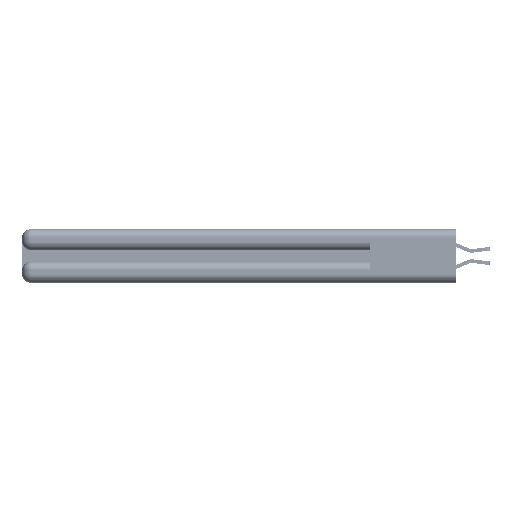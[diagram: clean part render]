
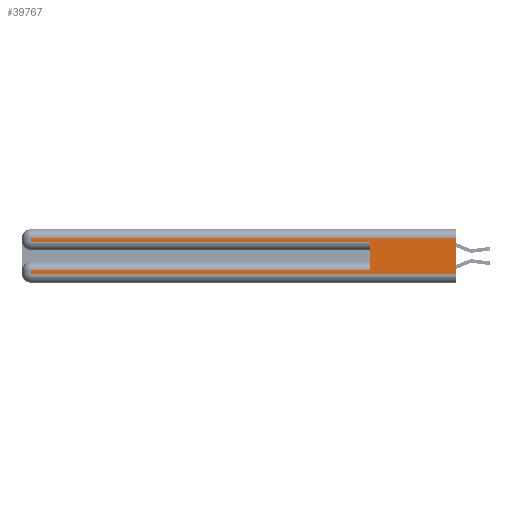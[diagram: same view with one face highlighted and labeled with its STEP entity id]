
A CAD part, left-side view. The second image highlights one B-rep face of the part: STEP entity #39767.
In plain terms, the highlighted planar face has unit normal (-1, 0, 0).
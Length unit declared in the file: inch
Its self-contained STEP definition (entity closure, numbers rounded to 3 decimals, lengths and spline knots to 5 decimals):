
#531 = ORIENTED_EDGE ( 'NONE', *, *, #10313, .T. ) ;
#702 = VERTEX_POINT ( 'NONE', #22128 ) ;
#866 = VECTOR ( 'NONE', #25597, 39.37008 ) ;
#1191 = CARTESIAN_POINT ( 'NONE',  ( 0., 0.6, 0.145 ) ) ;
#9027 = DIRECTION ( 'NONE',  ( 0., 1., 0. ) ) ;
#9532 = CARTESIAN_POINT ( 'NONE',  ( 0., 0.6, 0.085 ) ) ;
#10203 = LINE ( 'NONE', #1191, #27713 ) ;
#10313 = EDGE_CURVE ( 'NONE', #26561, #19253, #36068, .T. ) ;
#11097 = VECTOR ( 'NONE', #23661, 39.37008 ) ;
#11522 = EDGE_CURVE ( 'NONE', #47355, #26552, #30707, .T. ) ;
#12247 = ORIENTED_EDGE ( 'NONE', *, *, #44934, .T. ) ;
#12307 = EDGE_CURVE ( 'NONE', #19008, #36682, #10203, .T. ) ;
#14667 = DIRECTION ( 'NONE',  ( 0., 0., -1. ) ) ;
#15370 = LINE ( 'NONE', #38852, #42660 ) ;
#16777 = LINE ( 'NONE', #40078, #42897 ) ;
#17030 = DIRECTION ( 'NONE',  ( 0., 0., -1. ) ) ;
#18120 = CARTESIAN_POINT ( 'NONE',  ( 0., 2.94, 0.37 ) ) ;
#18336 = VECTOR ( 'NONE', #28219, 39.37008 ) ;
#18703 = ORIENTED_EDGE ( 'NONE', *, *, #11522, .T. ) ;
#19008 = VERTEX_POINT ( 'NONE', #9532 ) ;
#19253 = VERTEX_POINT ( 'NONE', #25702 ) ;
#19926 = CARTESIAN_POINT ( 'NONE',  ( 0., 0., 0.31 ) ) ;
#20222 = CARTESIAN_POINT ( 'NONE',  ( 0., 0., 0.31 ) ) ;
#20461 = ORIENTED_EDGE ( 'NONE', *, *, #26045, .T. ) ;
#22128 = CARTESIAN_POINT ( 'NONE',  ( 0., 0., 0.06 ) ) ;
#22239 = FACE_OUTER_BOUND ( 'NONE', #40934, .T. ) ;
#23595 = DIRECTION ( 'NONE',  ( 0., 0., 1. ) ) ;
#23661 = DIRECTION ( 'NONE',  ( 0., 1., 0. ) ) ;
#24463 = CARTESIAN_POINT ( 'NONE',  ( 0., 0., 0.285 ) ) ;
#25094 = ORIENTED_EDGE ( 'NONE', *, *, #31041, .F. ) ;
#25597 = DIRECTION ( 'NONE',  ( 0., 0., -1. ) ) ;
#25702 = CARTESIAN_POINT ( 'NONE',  ( 0., 2.94, 0.06 ) ) ;
#26031 = CARTESIAN_POINT ( 'NONE',  ( 0., 2.94, 0.37 ) ) ;
#26045 = EDGE_CURVE ( 'NONE', #19253, #702, #16777, .T. ) ;
#26552 = VERTEX_POINT ( 'NONE', #41825 ) ;
#26561 = VERTEX_POINT ( 'NONE', #27076 ) ;
#27076 = CARTESIAN_POINT ( 'NONE',  ( 0., 2.94, 0.085 ) ) ;
#27713 = VECTOR ( 'NONE', #23595, 39.37008 ) ;
#28219 = DIRECTION ( 'NONE',  ( 0., -1., 0. ) ) ;
#28240 = LINE ( 'NONE', #24463, #18336 ) ;
#29492 = PLANE ( 'NONE',  #30785 ) ;
#30132 = VECTOR ( 'NONE', #17030, 39.37008 ) ;
#30707 = LINE ( 'NONE', #18120, #866 ) ;
#30785 = AXIS2_PLACEMENT_3D ( 'NONE', #33253, #36964, #14667 ) ;
#31041 = EDGE_CURVE ( 'NONE', #31723, #702, #38812, .T. ) ;
#31723 = VERTEX_POINT ( 'NONE', #20222 ) ;
#33070 = EDGE_CURVE ( 'NONE', #19008, #26561, #15370, .T. ) ;
#33253 = CARTESIAN_POINT ( 'NONE',  ( 0., 0., 0.37 ) ) ;
#34906 = VECTOR ( 'NONE', #37090, 39.37008 ) ;
#36068 = LINE ( 'NONE', #26031, #34906 ) ;
#36682 = VERTEX_POINT ( 'NONE', #40381 ) ;
#36713 = CARTESIAN_POINT ( 'NONE',  ( 0., 2.94, 0.31 ) ) ;
#36964 = DIRECTION ( 'NONE',  ( 1., 0., 0. ) ) ;
#37090 = DIRECTION ( 'NONE',  ( 0., 0., -1. ) ) ;
#38812 = LINE ( 'NONE', #39288, #30132 ) ;
#38852 = CARTESIAN_POINT ( 'NONE',  ( 0., 0., 0.085 ) ) ;
#39288 = CARTESIAN_POINT ( 'NONE',  ( 0., 0., 0.37 ) ) ;
#39767 = ADVANCED_FACE ( 'NONE', ( #22239 ), #29492, .F. ) ;
#40078 = CARTESIAN_POINT ( 'NONE',  ( 0., 0., 0.06 ) ) ;
#40381 = CARTESIAN_POINT ( 'NONE',  ( 0., 0.6, 0.285 ) ) ;
#40812 = LINE ( 'NONE', #19926, #11097 ) ;
#40934 = EDGE_LOOP ( 'NONE', ( #25094, #44816, #18703, #12247, #44262, #45387, #531, #20461 ) ) ;
#41825 = CARTESIAN_POINT ( 'NONE',  ( 0., 2.94, 0.285 ) ) ;
#42660 = VECTOR ( 'NONE', #9027, 39.37008 ) ;
#42897 = VECTOR ( 'NONE', #47669, 39.37008 ) ;
#44262 = ORIENTED_EDGE ( 'NONE', *, *, #12307, .F. ) ;
#44816 = ORIENTED_EDGE ( 'NONE', *, *, #46610, .T. ) ;
#44934 = EDGE_CURVE ( 'NONE', #26552, #36682, #28240, .T. ) ;
#45387 = ORIENTED_EDGE ( 'NONE', *, *, #33070, .T. ) ;
#46610 = EDGE_CURVE ( 'NONE', #31723, #47355, #40812, .T. ) ;
#47355 = VERTEX_POINT ( 'NONE', #36713 ) ;
#47669 = DIRECTION ( 'NONE',  ( 0., -1., 0. ) ) ;
